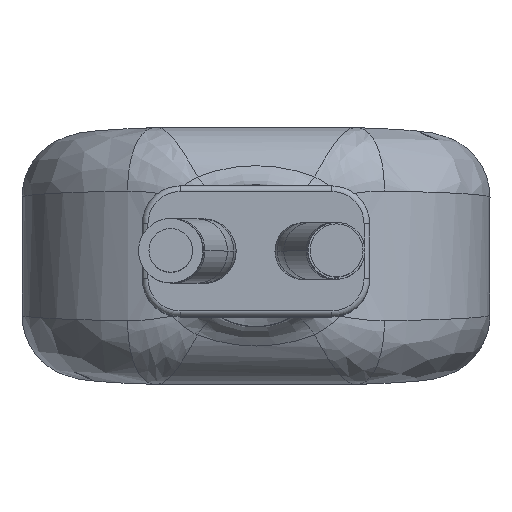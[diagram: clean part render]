
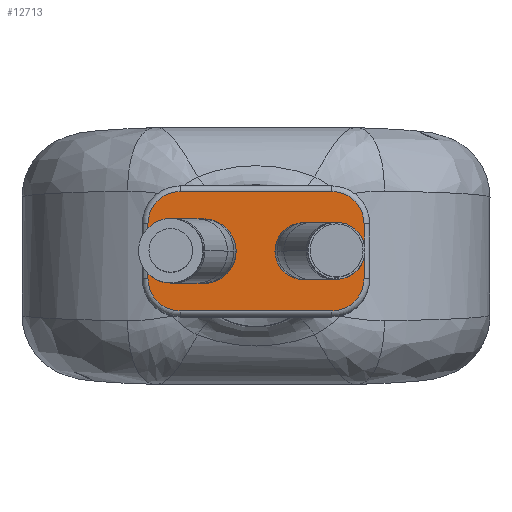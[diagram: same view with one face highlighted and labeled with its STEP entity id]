
A CAD part, top view. The second image highlights one B-rep face of the part: STEP entity #12713.
In plain terms, the highlighted planar face has unit normal (0, 0, 1).
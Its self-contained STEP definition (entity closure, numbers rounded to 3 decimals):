
#20 = EDGE_CURVE ( 'NONE', #14309, #10126, #4580, .T. ) ;
#101 = CARTESIAN_POINT ( 'NONE',  ( 5.7, 48.55, 172.5 ) ) ;
#182 = EDGE_CURVE ( 'NONE', #2167, #11285, #10801, .T. ) ;
#197 = ORIENTED_EDGE ( 'NONE', *, *, #8053, .T. ) ;
#484 = DIRECTION ( 'NONE',  ( 1., 0., 0. ) ) ;
#626 = CARTESIAN_POINT ( 'NONE',  ( -4.45, 50., 172.5 ) ) ;
#1002 = VERTEX_POINT ( 'NONE', #11570 ) ;
#1279 = LINE ( 'NONE', #14330, #8628 ) ;
#1303 = DIRECTION ( 'NONE',  ( 1., 0., 0. ) ) ;
#1331 = AXIS2_PLACEMENT_3D ( 'NONE', #13213, #12117, #1423 ) ;
#1423 = DIRECTION ( 'NONE',  ( 0., -1., 0. ) ) ;
#1592 = VECTOR ( 'NONE', #15422, 1000. ) ;
#1753 = EDGE_CURVE ( 'NONE', #11840, #3892, #15133, .T. ) ;
#2063 = CARTESIAN_POINT ( 'NONE',  ( -5.7, 48.55, 172.5 ) ) ;
#2121 = CIRCLE ( 'NONE', #14338, 1.7 ) ;
#2167 = VERTEX_POINT ( 'NONE', #4375 ) ;
#2224 = CARTESIAN_POINT ( 'NONE',  ( -1.05, 50., 172.5 ) ) ;
#2326 = CARTESIAN_POINT ( 'NONE',  ( 4., 51.45, 172.5 ) ) ;
#2703 = VERTEX_POINT ( 'NONE', #5130 ) ;
#2769 = EDGE_CURVE ( 'NONE', #10126, #14309, #4760, .T. ) ;
#2831 = DIRECTION ( 'NONE',  ( 0., 0., 1. ) ) ;
#2927 = ORIENTED_EDGE ( 'NONE', *, *, #9875, .T. ) ;
#3040 = DIRECTION ( 'NONE',  ( 1., 0., 0. ) ) ;
#3097 = ORIENTED_EDGE ( 'NONE', *, *, #15142, .T. ) ;
#3386 = AXIS2_PLACEMENT_3D ( 'NONE', #2326, #9429, #8356 ) ;
#3459 = EDGE_LOOP ( 'NONE', ( #2927, #6964, #7654, #4071, #12092, #3097, #197, #12089 ) ) ;
#3892 = VERTEX_POINT ( 'NONE', #10225 ) ;
#3945 = DIRECTION ( 'NONE',  ( 0., 0., 1. ) ) ;
#3965 = CARTESIAN_POINT ( 'NONE',  ( -5.7, 51.45, 172.5 ) ) ;
#4018 = CARTESIAN_POINT ( 'NONE',  ( 4., 53.15, 172.5 ) ) ;
#4071 = ORIENTED_EDGE ( 'NONE', *, *, #1753, .T. ) ;
#4294 = AXIS2_PLACEMENT_3D ( 'NONE', #8431, #13243, #1303 ) ;
#4372 = CIRCLE ( 'NONE', #3386, 1.7 ) ;
#4375 = CARTESIAN_POINT ( 'NONE',  ( 1., 50., 172.5 ) ) ;
#4580 = CIRCLE ( 'NONE', #12319, 1.7 ) ;
#4760 = CIRCLE ( 'NONE', #9999, 1.7 ) ;
#5130 = CARTESIAN_POINT ( 'NONE',  ( 5.7, 51.45, 172.5 ) ) ;
#5233 = VECTOR ( 'NONE', #12394, 1000. ) ;
#5432 = CARTESIAN_POINT ( 'NONE',  ( -4., 53.15, 172.5 ) ) ;
#5619 = FACE_BOUND ( 'NONE', #13859, .T. ) ;
#6063 = CIRCLE ( 'NONE', #4294, 1.5 ) ;
#6119 = DIRECTION ( 'NONE',  ( 1., 0., 0. ) ) ;
#6143 = DIRECTION ( 'NONE',  ( 0., 1., 0. ) ) ;
#6397 = CARTESIAN_POINT ( 'NONE',  ( -4., 48.55, 172.5 ) ) ;
#6845 = ORIENTED_EDGE ( 'NONE', *, *, #182, .T. ) ;
#6848 = VECTOR ( 'NONE', #11987, 1000. ) ;
#6964 = ORIENTED_EDGE ( 'NONE', *, *, #7774, .T. ) ;
#7001 = AXIS2_PLACEMENT_3D ( 'NONE', #8781, #2831, #484 ) ;
#7654 = ORIENTED_EDGE ( 'NONE', *, *, #12333, .T. ) ;
#7774 = EDGE_CURVE ( 'NONE', #10404, #11226, #1279, .T. ) ;
#7986 = FACE_OUTER_BOUND ( 'NONE', #3459, .T. ) ;
#8036 = DIRECTION ( 'NONE',  ( 0., 0., -1. ) ) ;
#8053 = EDGE_CURVE ( 'NONE', #2703, #14044, #4372, .T. ) ;
#8356 = DIRECTION ( 'NONE',  ( 1., 0., 0. ) ) ;
#8401 = DIRECTION ( 'NONE',  ( 0., 0., -1. ) ) ;
#8431 = CARTESIAN_POINT ( 'NONE',  ( 2.5, 50., 172.5 ) ) ;
#8628 = VECTOR ( 'NONE', #8913, 1000. ) ;
#8763 = VERTEX_POINT ( 'NONE', #5432 ) ;
#8781 = CARTESIAN_POINT ( 'NONE',  ( 0., 50., 172.5 ) ) ;
#8852 = PLANE ( 'NONE',  #7001 ) ;
#8866 = AXIS2_PLACEMENT_3D ( 'NONE', #6397, #14013, #9252 ) ;
#8913 = DIRECTION ( 'NONE',  ( 0., -1., 0. ) ) ;
#8996 = CARTESIAN_POINT ( 'NONE',  ( 2.5, 50., 172.5 ) ) ;
#9053 = AXIS2_PLACEMENT_3D ( 'NONE', #8996, #13746, #3040 ) ;
#9201 = CARTESIAN_POINT ( 'NONE',  ( -4., 46.85, 172.5 ) ) ;
#9252 = DIRECTION ( 'NONE',  ( -1., 0., 0. ) ) ;
#9260 = EDGE_CURVE ( 'NONE', #3892, #1002, #13038, .T. ) ;
#9360 = ORIENTED_EDGE ( 'NONE', *, *, #2769, .T. ) ;
#9429 = DIRECTION ( 'NONE',  ( 0., 0., 1. ) ) ;
#9875 = EDGE_CURVE ( 'NONE', #8763, #10404, #2121, .T. ) ;
#9999 = AXIS2_PLACEMENT_3D ( 'NONE', #12684, #8036, #12605 ) ;
#10126 = VERTEX_POINT ( 'NONE', #626 ) ;
#10225 = CARTESIAN_POINT ( 'NONE',  ( 4., 46.85, 172.5 ) ) ;
#10404 = VERTEX_POINT ( 'NONE', #3965 ) ;
#10652 = ORIENTED_EDGE ( 'NONE', *, *, #20, .T. ) ;
#10801 = CIRCLE ( 'NONE', #9053, 1.5 ) ;
#11226 = VERTEX_POINT ( 'NONE', #2063 ) ;
#11285 = VERTEX_POINT ( 'NONE', #14554 ) ;
#11293 = EDGE_LOOP ( 'NONE', ( #9360, #10652 ) ) ;
#11570 = CARTESIAN_POINT ( 'NONE',  ( 5.7, 48.55, 172.5 ) ) ;
#11664 = CARTESIAN_POINT ( 'NONE',  ( -4., 46.85, 172.5 ) ) ;
#11759 = EDGE_CURVE ( 'NONE', #14044, #8763, #12219, .T. ) ;
#11840 = VERTEX_POINT ( 'NONE', #11664 ) ;
#11905 = CARTESIAN_POINT ( 'NONE',  ( 4., 53.15, 172.5 ) ) ;
#11987 = DIRECTION ( 'NONE',  ( -1., 0., 0. ) ) ;
#12089 = ORIENTED_EDGE ( 'NONE', *, *, #11759, .T. ) ;
#12092 = ORIENTED_EDGE ( 'NONE', *, *, #9260, .T. ) ;
#12117 = DIRECTION ( 'NONE',  ( 0., 0., 1. ) ) ;
#12130 = LINE ( 'NONE', #101, #1592 ) ;
#12219 = LINE ( 'NONE', #4018, #6848 ) ;
#12319 = AXIS2_PLACEMENT_3D ( 'NONE', #13368, #8401, #6119 ) ;
#12333 = EDGE_CURVE ( 'NONE', #11226, #11840, #15100, .T. ) ;
#12394 = DIRECTION ( 'NONE',  ( 1., 0., 0. ) ) ;
#12605 = DIRECTION ( 'NONE',  ( 1., 0., 0. ) ) ;
#12684 = CARTESIAN_POINT ( 'NONE',  ( -2.75, 50., 172.5 ) ) ;
#12713 = ADVANCED_FACE ( 'NONE', ( #7986, #5619, #14861 ), #8852, .T. ) ;
#13038 = CIRCLE ( 'NONE', #1331, 1.7 ) ;
#13213 = CARTESIAN_POINT ( 'NONE',  ( 4., 48.55, 172.5 ) ) ;
#13225 = ORIENTED_EDGE ( 'NONE', *, *, #14776, .T. ) ;
#13243 = DIRECTION ( 'NONE',  ( 0., 0., -1. ) ) ;
#13368 = CARTESIAN_POINT ( 'NONE',  ( -2.75, 50., 172.5 ) ) ;
#13746 = DIRECTION ( 'NONE',  ( 0., 0., -1. ) ) ;
#13859 = EDGE_LOOP ( 'NONE', ( #6845, #13225 ) ) ;
#14013 = DIRECTION ( 'NONE',  ( 0., 0., 1. ) ) ;
#14044 = VERTEX_POINT ( 'NONE', #11905 ) ;
#14309 = VERTEX_POINT ( 'NONE', #2224 ) ;
#14330 = CARTESIAN_POINT ( 'NONE',  ( -5.7, 51.45, 172.5 ) ) ;
#14338 = AXIS2_PLACEMENT_3D ( 'NONE', #14661, #3945, #6143 ) ;
#14554 = CARTESIAN_POINT ( 'NONE',  ( 4., 50., 172.5 ) ) ;
#14661 = CARTESIAN_POINT ( 'NONE',  ( -4., 51.45, 172.5 ) ) ;
#14776 = EDGE_CURVE ( 'NONE', #11285, #2167, #6063, .T. ) ;
#14861 = FACE_BOUND ( 'NONE', #11293, .T. ) ;
#15100 = CIRCLE ( 'NONE', #8866, 1.7 ) ;
#15133 = LINE ( 'NONE', #9201, #5233 ) ;
#15142 = EDGE_CURVE ( 'NONE', #1002, #2703, #12130, .T. ) ;
#15422 = DIRECTION ( 'NONE',  ( 0., 1., 0. ) ) ;
